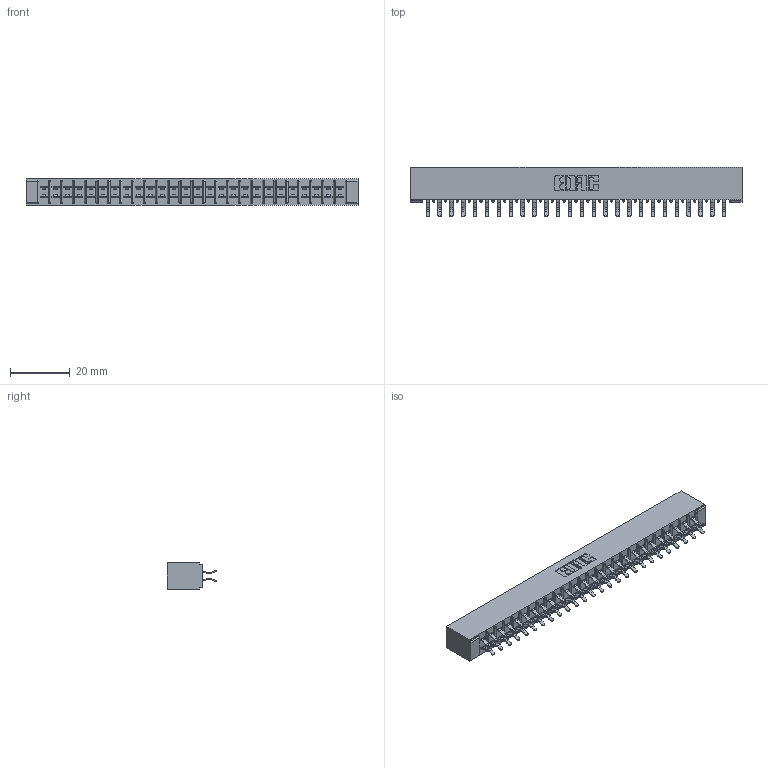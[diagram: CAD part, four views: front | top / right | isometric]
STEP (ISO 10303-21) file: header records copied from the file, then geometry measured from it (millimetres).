
FILE_DESCRIPTION (( 'STEP AP203' ), '1' );
FILE_NAME ('305-052-556-201.STEP', '2019-09-09T22:36:21', ( '' ), ( '' ), 'SwSTEP 2.0', 'SolidWorks 2016', '' );
FILE_SCHEMA (( 'CONFIG_CONTROL_DESIGN' ));
Length unit declared in the file: inch
Products named in the file (3): 305-052-556-201; 305-290-001_556; 305 Part_No Mounting
Assembly tree (53 placements, depth 2):
  305-052-556-201
    305 Part_No Mounting
    305-290-001_556  x52
Bounding box: 110.9 x 16.64 x 8.71 mm (x, y, z)
Volume: 7127.8 mm3; surface area: 14289.9 mm2
Topology: 53 solids, 53 shells, 3020 faces, 8690 edges, 5652 vertices
Faces by surface type: plane 1676, cylinder 1240, sphere 104
Entity records: 30043 total; most frequent: CARTESIAN_POINT 4972, ORIENTED_EDGE 4932, DIRECTION 4824, EDGE_CURVE 2466, VECTOR 1976, LINE 1976, VERTEX_POINT 1572, AXIS2_PLACEMENT_3D 1424
